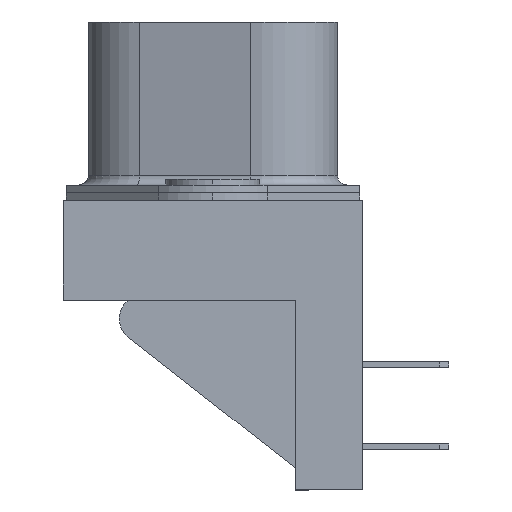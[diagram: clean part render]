
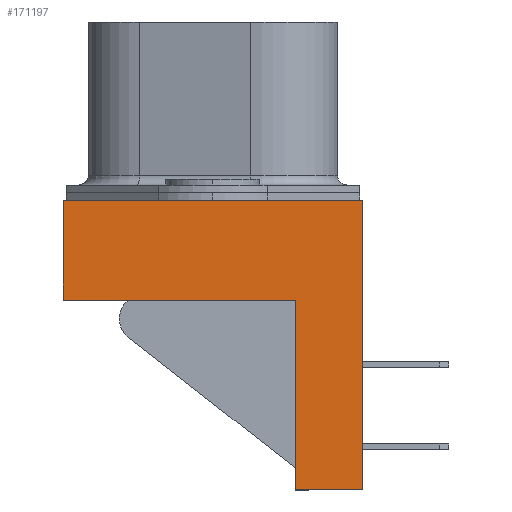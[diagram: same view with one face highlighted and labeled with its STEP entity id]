
A CAD part, left-side view. The second image highlights one B-rep face of the part: STEP entity #171197.
In plain terms, the highlighted planar face has unit normal (-1, 0, 0).
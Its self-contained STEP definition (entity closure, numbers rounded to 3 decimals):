
#3294 = EDGE_CURVE ( 'NONE', #104057, #171035, #106594, .T. ) ;
#12094 = DIRECTION ( 'NONE',  ( 0., -1., 0. ) ) ;
#18110 = VERTEX_POINT ( 'NONE', #83306 ) ;
#22075 = CARTESIAN_POINT ( 'NONE',  ( -4.125, -4.3, -15.1 ) ) ;
#26685 = VECTOR ( 'NONE', #74353, 1000. ) ;
#27050 = PLANE ( 'NONE',  #94937 ) ;
#28808 = DIRECTION ( 'NONE',  ( 0., -1., 0. ) ) ;
#29852 = VECTOR ( 'NONE', #149563, 1000. ) ;
#31858 = EDGE_CURVE ( 'NONE', #119195, #88200, #52275, .T. ) ;
#32589 = EDGE_CURVE ( 'NONE', #171035, #119195, #48349, .T. ) ;
#34967 = DIRECTION ( 'NONE',  ( 0., 0., 1. ) ) ;
#37828 = ORIENTED_EDGE ( 'NONE', *, *, #31858, .F. ) ;
#46714 = LINE ( 'NONE', #142137, #26685 ) ;
#48349 = LINE ( 'NONE', #128659, #173388 ) ;
#50423 = DIRECTION ( 'NONE',  ( 0., 1., 0. ) ) ;
#50627 = LINE ( 'NONE', #22075, #29852 ) ;
#52275 = LINE ( 'NONE', #119206, #138977 ) ;
#54745 = LINE ( 'NONE', #110057, #173867 ) ;
#56468 = CARTESIAN_POINT ( 'NONE',  ( -4.125, 7.8, -15.1 ) ) ;
#64077 = ORIENTED_EDGE ( 'NONE', *, *, #81224, .T. ) ;
#70783 = CARTESIAN_POINT ( 'NONE',  ( -4.125, -7.8, 0. ) ) ;
#72432 = ORIENTED_EDGE ( 'NONE', *, *, #32589, .F. ) ;
#73300 = CARTESIAN_POINT ( 'NONE',  ( -4.125, -4.3, -15.1 ) ) ;
#74353 = DIRECTION ( 'NONE',  ( 0., -1., 0. ) ) ;
#79706 = EDGE_LOOP ( 'NONE', ( #109181, #81102, #107386, #64077, #37828, #72432 ) ) ;
#80610 = CARTESIAN_POINT ( 'NONE',  ( -4.125, 7.8, -5.2 ) ) ;
#81102 = ORIENTED_EDGE ( 'NONE', *, *, #172917, .F. ) ;
#81224 = EDGE_CURVE ( 'NONE', #18110, #88200, #54745, .T. ) ;
#83306 = CARTESIAN_POINT ( 'NONE',  ( -4.125, -7.8, -15.1 ) ) ;
#88200 = VERTEX_POINT ( 'NONE', #70783 ) ;
#90224 = EDGE_CURVE ( 'NONE', #132447, #18110, #46714, .T. ) ;
#94937 = AXIS2_PLACEMENT_3D ( 'NONE', #56468, #166207, #28808 ) ;
#104057 = VERTEX_POINT ( 'NONE', #160399 ) ;
#106594 = LINE ( 'NONE', #173524, #118569 ) ;
#107386 = ORIENTED_EDGE ( 'NONE', *, *, #90224, .T. ) ;
#107435 = DIRECTION ( 'NONE',  ( 0., 0., 1. ) ) ;
#109181 = ORIENTED_EDGE ( 'NONE', *, *, #3294, .F. ) ;
#110057 = CARTESIAN_POINT ( 'NONE',  ( -4.125, -7.8, -15.1 ) ) ;
#118569 = VECTOR ( 'NONE', #50423, 1000. ) ;
#119195 = VERTEX_POINT ( 'NONE', #163028 ) ;
#119206 = CARTESIAN_POINT ( 'NONE',  ( -4.125, 7.8, 0. ) ) ;
#128659 = CARTESIAN_POINT ( 'NONE',  ( -4.125, 7.8, -15.1 ) ) ;
#132447 = VERTEX_POINT ( 'NONE', #73300 ) ;
#135905 = FACE_OUTER_BOUND ( 'NONE', #79706, .T. ) ;
#138977 = VECTOR ( 'NONE', #12094, 1000. ) ;
#142137 = CARTESIAN_POINT ( 'NONE',  ( -4.125, 7.8, -15.1 ) ) ;
#149563 = DIRECTION ( 'NONE',  ( 0., 0., 1. ) ) ;
#160399 = CARTESIAN_POINT ( 'NONE',  ( -4.125, -4.3, -5.2 ) ) ;
#163028 = CARTESIAN_POINT ( 'NONE',  ( -4.125, 7.8, 0. ) ) ;
#166207 = DIRECTION ( 'NONE',  ( -1., 0., 0. ) ) ;
#171035 = VERTEX_POINT ( 'NONE', #80610 ) ;
#171197 = ADVANCED_FACE ( 'NONE', ( #135905 ), #27050, .T. ) ;
#172917 = EDGE_CURVE ( 'NONE', #132447, #104057, #50627, .T. ) ;
#173388 = VECTOR ( 'NONE', #34967, 1000. ) ;
#173524 = CARTESIAN_POINT ( 'NONE',  ( -4.125, 7.8, -5.2 ) ) ;
#173867 = VECTOR ( 'NONE', #107435, 1000. ) ;
